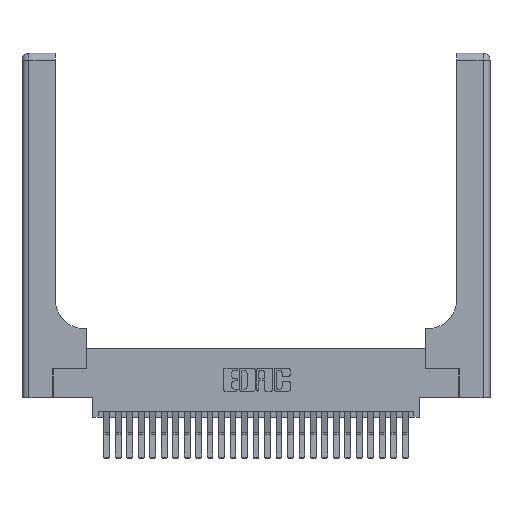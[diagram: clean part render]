
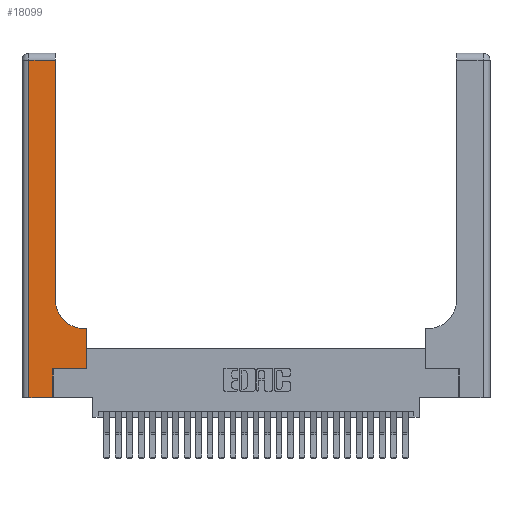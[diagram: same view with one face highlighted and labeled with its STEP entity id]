
A CAD part, top view. The second image highlights one B-rep face of the part: STEP entity #18099.
In plain terms, the highlighted planar face has unit normal (0, 0, 1).
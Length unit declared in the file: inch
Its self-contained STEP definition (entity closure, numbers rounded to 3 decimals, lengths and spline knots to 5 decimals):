
#93 = CARTESIAN_POINT ( 'NONE',  ( 0.269, 0.25, 0.37 ) ) ;
#121 = PLANE ( 'NONE',  #19325 ) ;
#143 = EDGE_CURVE ( 'NONE', #24359, #13648, #17679, .T. ) ;
#528 = VERTEX_POINT ( 'NONE', #18668 ) ;
#583 = CARTESIAN_POINT ( 'NONE',  ( 0.2915, 0.6, 0.37 ) ) ;
#607 = ORIENTED_EDGE ( 'NONE', *, *, #766, .T. ) ;
#766 = EDGE_CURVE ( 'NONE', #15093, #962, #3051, .T. ) ;
#962 = VERTEX_POINT ( 'NONE', #9390 ) ;
#2178 = EDGE_CURVE ( 'NONE', #528, #7049, #17569, .T. ) ;
#2483 = DIRECTION ( 'NONE',  ( 1., 0., 0. ) ) ;
#2509 = DIRECTION ( 'NONE',  ( 0., 0., -1. ) ) ;
#3051 = LINE ( 'NONE', #13727, #25767 ) ;
#3859 = ORIENTED_EDGE ( 'NONE', *, *, #11395, .T. ) ;
#4225 = ORIENTED_EDGE ( 'NONE', *, *, #22502, .T. ) ;
#4797 = VECTOR ( 'NONE', #25029, 39.37008 ) ;
#5100 = VECTOR ( 'NONE', #26683, 39.37008 ) ;
#5316 = CARTESIAN_POINT ( 'NONE',  ( 0.06, 2.94, 0.37 ) ) ;
#6687 = VERTEX_POINT ( 'NONE', #10343 ) ;
#7049 = VERTEX_POINT ( 'NONE', #22187 ) ;
#7087 = EDGE_CURVE ( 'NONE', #6687, #14016, #7976, .T. ) ;
#7410 = VECTOR ( 'NONE', #14115, 39.37008 ) ;
#7976 = LINE ( 'NONE', #93, #18897 ) ;
#8140 = FACE_OUTER_BOUND ( 'NONE', #13679, .T. ) ;
#8594 = ORIENTED_EDGE ( 'NONE', *, *, #12636, .T. ) ;
#9390 = CARTESIAN_POINT ( 'NONE',  ( 0.2915, 2.94, 0.37 ) ) ;
#9923 = CARTESIAN_POINT ( 'NONE',  ( 0., 0., 0.37 ) ) ;
#10118 = ORIENTED_EDGE ( 'NONE', *, *, #14520, .T. ) ;
#10343 = CARTESIAN_POINT ( 'NONE',  ( 0.269, 0.25, 0.37 ) ) ;
#10471 = CARTESIAN_POINT ( 'NONE',  ( 0.5415, 0.85, 0.37 ) ) ;
#11292 = VECTOR ( 'NONE', #12910, 39.37008 ) ;
#11395 = EDGE_CURVE ( 'NONE', #13648, #26435, #24781, .T. ) ;
#12550 = VECTOR ( 'NONE', #27635, 39.37008 ) ;
#12631 = DIRECTION ( 'NONE',  ( 1., 0., 0. ) ) ;
#12636 = EDGE_CURVE ( 'NONE', #962, #24359, #17286, .T. ) ;
#12910 = DIRECTION ( 'NONE',  ( 0., 1., 0. ) ) ;
#13648 = VERTEX_POINT ( 'NONE', #20247 ) ;
#13679 = EDGE_LOOP ( 'NONE', ( #607, #8594, #26305, #3859, #24707, #18013, #10118, #18448, #4225 ) ) ;
#13697 = DIRECTION ( 'NONE',  ( 0., 1., 0. ) ) ;
#13727 = CARTESIAN_POINT ( 'NONE',  ( 0.2915, 3., 0.37 ) ) ;
#14016 = VERTEX_POINT ( 'NONE', #15033 ) ;
#14115 = DIRECTION ( 'NONE',  ( 1., 0., 0. ) ) ;
#14520 = EDGE_CURVE ( 'NONE', #14016, #528, #23248, .T. ) ;
#15033 = CARTESIAN_POINT ( 'NONE',  ( 0.5585, 0.25, 0.37 ) ) ;
#15093 = VERTEX_POINT ( 'NONE', #16684 ) ;
#15897 = CARTESIAN_POINT ( 'NONE',  ( 0., 3., 0.37 ) ) ;
#16684 = CARTESIAN_POINT ( 'NONE',  ( 0.2915, 0.85, 0.37 ) ) ;
#17077 = LINE ( 'NONE', #19400, #11292 ) ;
#17286 = LINE ( 'NONE', #22827, #4797 ) ;
#17569 = LINE ( 'NONE', #583, #5100 ) ;
#17679 = LINE ( 'NONE', #28028, #12550 ) ;
#18013 = ORIENTED_EDGE ( 'NONE', *, *, #7087, .T. ) ;
#18055 = DIRECTION ( 'NONE',  ( -1., 0., 0. ) ) ;
#18099 = ADVANCED_FACE ( 'NONE', ( #8140 ), #121, .F. ) ;
#18448 = ORIENTED_EDGE ( 'NONE', *, *, #2178, .T. ) ;
#18668 = CARTESIAN_POINT ( 'NONE',  ( 0.5585, 0.6, 0.37 ) ) ;
#18897 = VECTOR ( 'NONE', #2483, 39.37008 ) ;
#19142 = CARTESIAN_POINT ( 'NONE',  ( 0.5585, 0.25, 0.37 ) ) ;
#19325 = AXIS2_PLACEMENT_3D ( 'NONE', #15897, #2509, #18055 ) ;
#19400 = CARTESIAN_POINT ( 'NONE',  ( 0.269, 0., 0.37 ) ) ;
#19734 = CARTESIAN_POINT ( 'NONE',  ( 0.269, 0., 0.37 ) ) ;
#20247 = CARTESIAN_POINT ( 'NONE',  ( 0.06, 0., 0.37 ) ) ;
#20803 = EDGE_CURVE ( 'NONE', #26435, #6687, #17077, .T. ) ;
#21917 = VECTOR ( 'NONE', #23464, 39.37008 ) ;
#22187 = CARTESIAN_POINT ( 'NONE',  ( 0.5415, 0.6, 0.37 ) ) ;
#22502 = EDGE_CURVE ( 'NONE', #7049, #15093, #26102, .T. ) ;
#22827 = CARTESIAN_POINT ( 'NONE',  ( 0., 2.94, 0.37 ) ) ;
#23248 = LINE ( 'NONE', #19142, #21917 ) ;
#23464 = DIRECTION ( 'NONE',  ( 0., 1., 0. ) ) ;
#24359 = VERTEX_POINT ( 'NONE', #5316 ) ;
#24707 = ORIENTED_EDGE ( 'NONE', *, *, #20803, .T. ) ;
#24781 = LINE ( 'NONE', #9923, #7410 ) ;
#25029 = DIRECTION ( 'NONE',  ( -1., 0., 0. ) ) ;
#25642 = DIRECTION ( 'NONE',  ( 0., 0., -1. ) ) ;
#25767 = VECTOR ( 'NONE', #13697, 39.37008 ) ;
#26102 = CIRCLE ( 'NONE', #26154, 0.25 ) ;
#26154 = AXIS2_PLACEMENT_3D ( 'NONE', #10471, #25642, #12631 ) ;
#26305 = ORIENTED_EDGE ( 'NONE', *, *, #143, .T. ) ;
#26435 = VERTEX_POINT ( 'NONE', #19734 ) ;
#26683 = DIRECTION ( 'NONE',  ( -1., 0., 0. ) ) ;
#27635 = DIRECTION ( 'NONE',  ( 0., -1., 0. ) ) ;
#28028 = CARTESIAN_POINT ( 'NONE',  ( 0.06, 3., 0.37 ) ) ;
